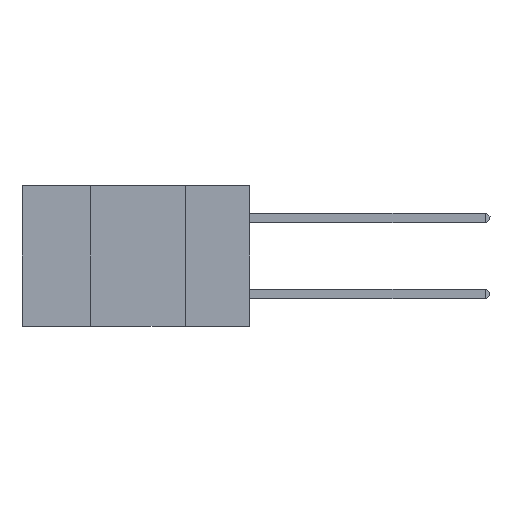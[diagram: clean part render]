
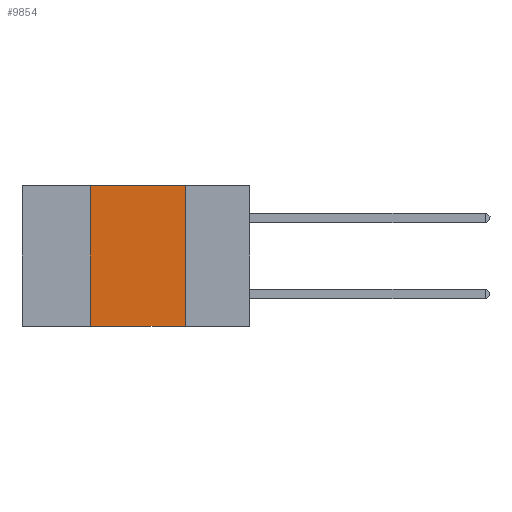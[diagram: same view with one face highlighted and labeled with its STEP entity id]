
A CAD part, left-side view. The second image highlights one B-rep face of the part: STEP entity #9854.
In plain terms, the highlighted planar face has unit normal (-1, 0, 0).
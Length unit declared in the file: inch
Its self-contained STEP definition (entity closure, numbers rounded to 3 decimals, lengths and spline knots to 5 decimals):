
#120 = DIRECTION ( 'NONE',  ( 0., 0., 1. ) ) ;
#316 = DIRECTION ( 'NONE',  ( 0., 0., -1. ) ) ;
#385 = CARTESIAN_POINT ( 'NONE',  ( 0., 0.17, 0. ) ) ;
#543 = AXIS2_PLACEMENT_3D ( 'NONE', #9213, #5893, #12471 ) ;
#918 = VECTOR ( 'NONE', #10538, 39.37008 ) ;
#1005 = VERTEX_POINT ( 'NONE', #6608 ) ;
#1555 = EDGE_LOOP ( 'NONE', ( #13507, #11167, #3341, #12136 ) ) ;
#1569 = PLANE ( 'NONE',  #543 ) ;
#1957 = LINE ( 'NONE', #2173, #5232 ) ;
#2057 = VECTOR ( 'NONE', #2885, 39.37008 ) ;
#2173 = CARTESIAN_POINT ( 'NONE',  ( 0., 0.42, 0. ) ) ;
#2235 = VECTOR ( 'NONE', #316, 39.37008 ) ;
#2885 = DIRECTION ( 'NONE',  ( 0., -1., 0. ) ) ;
#2942 = EDGE_CURVE ( 'NONE', #6815, #5407, #3576, .T. ) ;
#3341 = ORIENTED_EDGE ( 'NONE', *, *, #3410, .F. ) ;
#3410 = EDGE_CURVE ( 'NONE', #1005, #6815, #1957, .T. ) ;
#3414 = LINE ( 'NONE', #9933, #2235 ) ;
#3576 = LINE ( 'NONE', #8362, #2057 ) ;
#3720 = CARTESIAN_POINT ( 'NONE',  ( 0., 0.42, 0. ) ) ;
#4950 = CARTESIAN_POINT ( 'NONE',  ( 0., 0.6, -0.37 ) ) ;
#5232 = VECTOR ( 'NONE', #120, 39.37008 ) ;
#5407 = VERTEX_POINT ( 'NONE', #385 ) ;
#5893 = DIRECTION ( 'NONE',  ( 1., 0., 0. ) ) ;
#6608 = CARTESIAN_POINT ( 'NONE',  ( 0., 0.42, -0.37 ) ) ;
#6815 = VERTEX_POINT ( 'NONE', #3720 ) ;
#8362 = CARTESIAN_POINT ( 'NONE',  ( 0., 0.6, 0. ) ) ;
#9213 = CARTESIAN_POINT ( 'NONE',  ( 0., 0.6, 0. ) ) ;
#9854 = ADVANCED_FACE ( 'NONE', ( #13951 ), #1569, .F. ) ;
#9933 = CARTESIAN_POINT ( 'NONE',  ( 0., 0.17, 0. ) ) ;
#10538 = DIRECTION ( 'NONE',  ( 0., -1., 0. ) ) ;
#11167 = ORIENTED_EDGE ( 'NONE', *, *, #2942, .F. ) ;
#11376 = CARTESIAN_POINT ( 'NONE',  ( 0., 0.17, -0.37 ) ) ;
#12136 = ORIENTED_EDGE ( 'NONE', *, *, #12597, .T. ) ;
#12471 = DIRECTION ( 'NONE',  ( 0., 0., -1. ) ) ;
#12597 = EDGE_CURVE ( 'NONE', #1005, #12660, #12821, .T. ) ;
#12660 = VERTEX_POINT ( 'NONE', #11376 ) ;
#12821 = LINE ( 'NONE', #4950, #918 ) ;
#12924 = EDGE_CURVE ( 'NONE', #5407, #12660, #3414, .T. ) ;
#13507 = ORIENTED_EDGE ( 'NONE', *, *, #12924, .F. ) ;
#13951 = FACE_OUTER_BOUND ( 'NONE', #1555, .T. ) ;
